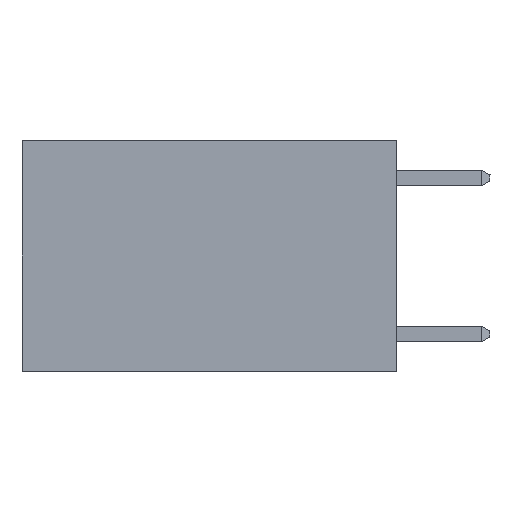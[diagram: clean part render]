
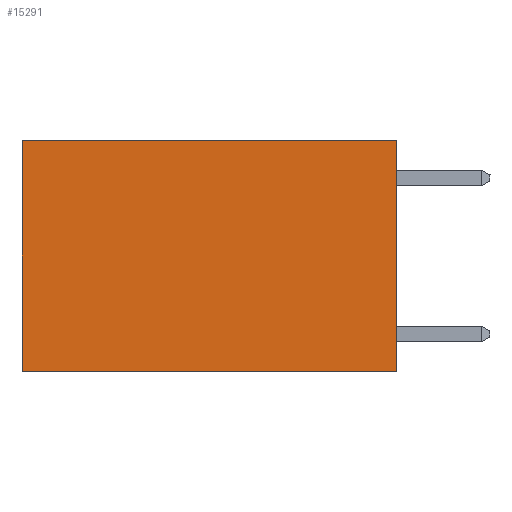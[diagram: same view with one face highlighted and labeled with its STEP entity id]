
A CAD part, left-side view. The second image highlights one B-rep face of the part: STEP entity #15291.
In plain terms, the highlighted planar face has unit normal (-1, 0, 0).
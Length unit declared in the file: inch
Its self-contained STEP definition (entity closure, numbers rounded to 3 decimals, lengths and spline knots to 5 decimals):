
#23 = CARTESIAN_POINT ( 'NONE',  ( 0.2625, 0.6, 0. ) ) ;
#1030 = DIRECTION ( 'NONE',  ( 0., 1., 0. ) ) ;
#1645 = VECTOR ( 'NONE', #1030, 39.37008 ) ;
#1830 = ORIENTED_EDGE ( 'NONE', *, *, #6681, .T. ) ;
#2509 = LINE ( 'NONE', #5086, #1645 ) ;
#3154 = EDGE_CURVE ( 'NONE', #13736, #8504, #15670, .T. ) ;
#3339 = CARTESIAN_POINT ( 'NONE',  ( 0.2625, 0.6, 0. ) ) ;
#3546 = DIRECTION ( 'NONE',  ( 0., 0., -1. ) ) ;
#3730 = CARTESIAN_POINT ( 'NONE',  ( 0.2625, 0., 0. ) ) ;
#3799 = EDGE_CURVE ( 'NONE', #8504, #4138, #2509, .T. ) ;
#4138 = VERTEX_POINT ( 'NONE', #12408 ) ;
#4475 = VECTOR ( 'NONE', #10140, 39.37008 ) ;
#5013 = FACE_OUTER_BOUND ( 'NONE', #16439, .T. ) ;
#5086 = CARTESIAN_POINT ( 'NONE',  ( 0.2625, 0., -0.37 ) ) ;
#5093 = VECTOR ( 'NONE', #3546, 39.37008 ) ;
#5793 = DIRECTION ( 'NONE',  ( 0., 0., -1. ) ) ;
#6472 = DIRECTION ( 'NONE',  ( 0., 1., 0. ) ) ;
#6681 = EDGE_CURVE ( 'NONE', #15825, #4138, #15089, .T. ) ;
#6783 = CARTESIAN_POINT ( 'NONE',  ( 0.2625, 0., 0. ) ) ;
#7502 = EDGE_CURVE ( 'NONE', #13736, #15825, #15287, .T. ) ;
#8433 = CARTESIAN_POINT ( 'NONE',  ( 0.2625, 0., -0.37 ) ) ;
#8504 = VERTEX_POINT ( 'NONE', #8433 ) ;
#8698 = AXIS2_PLACEMENT_3D ( 'NONE', #9782, #13758, #5793 ) ;
#9064 = ORIENTED_EDGE ( 'NONE', *, *, #3799, .F. ) ;
#9782 = CARTESIAN_POINT ( 'NONE',  ( 0.2625, 0., 0. ) ) ;
#10140 = DIRECTION ( 'NONE',  ( 0., 0., -1. ) ) ;
#12408 = CARTESIAN_POINT ( 'NONE',  ( 0.2625, 0.6, -0.37 ) ) ;
#12454 = PLANE ( 'NONE',  #8698 ) ;
#12929 = CARTESIAN_POINT ( 'NONE',  ( 0.2625, 0., 0. ) ) ;
#12983 = ORIENTED_EDGE ( 'NONE', *, *, #7502, .T. ) ;
#13736 = VERTEX_POINT ( 'NONE', #6783 ) ;
#13758 = DIRECTION ( 'NONE',  ( 1., 0., 0. ) ) ;
#14062 = VECTOR ( 'NONE', #6472, 39.37008 ) ;
#15089 = LINE ( 'NONE', #3339, #4475 ) ;
#15287 = LINE ( 'NONE', #3730, #14062 ) ;
#15291 = ADVANCED_FACE ( 'NONE', ( #5013 ), #12454, .F. ) ;
#15670 = LINE ( 'NONE', #12929, #5093 ) ;
#15825 = VERTEX_POINT ( 'NONE', #23 ) ;
#16044 = ORIENTED_EDGE ( 'NONE', *, *, #3154, .F. ) ;
#16439 = EDGE_LOOP ( 'NONE', ( #1830, #9064, #16044, #12983 ) ) ;
